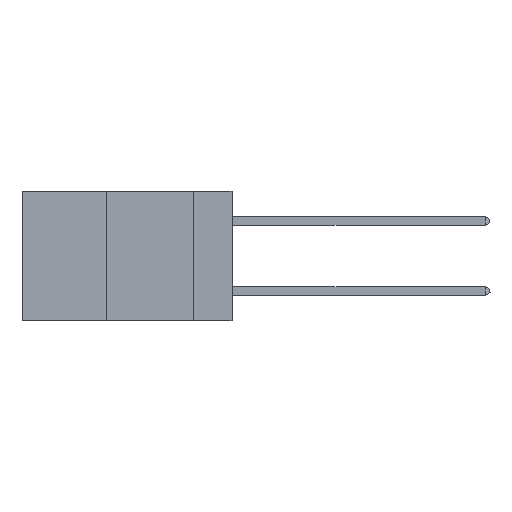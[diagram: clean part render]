
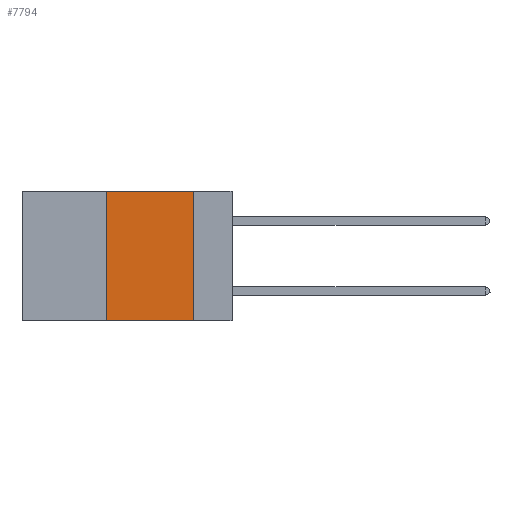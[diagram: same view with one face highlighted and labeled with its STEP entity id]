
A CAD part, left-side view. The second image highlights one B-rep face of the part: STEP entity #7794.
In plain terms, the highlighted planar face has unit normal (-1, 0, 0).
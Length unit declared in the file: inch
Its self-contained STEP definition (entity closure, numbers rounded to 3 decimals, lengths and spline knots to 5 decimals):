
#4075 = VERTEX_POINT ( 'NONE', #21904 ) ;
#4447 = VECTOR ( 'NONE', #21325, 39.37008 ) ;
#6490 = EDGE_CURVE ( 'NONE', #4075, #15165, #25839, .T. ) ;
#7478 = VECTOR ( 'NONE', #22442, 39.37008 ) ;
#7794 = ADVANCED_FACE ( 'NONE', ( #26321 ), #20868, .F. ) ;
#9089 = ORIENTED_EDGE ( 'NONE', *, *, #14328, .T. ) ;
#9822 = CARTESIAN_POINT ( 'NONE',  ( 0., 0.11, -0.37 ) ) ;
#9927 = CARTESIAN_POINT ( 'NONE',  ( 0., 0.11, 0. ) ) ;
#10688 = AXIS2_PLACEMENT_3D ( 'NONE', #18592, #23290, #18900 ) ;
#11420 = CARTESIAN_POINT ( 'NONE',  ( 0., 0.11, 0. ) ) ;
#12205 = LINE ( 'NONE', #24849, #7478 ) ;
#12572 = VECTOR ( 'NONE', #28287, 39.37008 ) ;
#12920 = LINE ( 'NONE', #17652, #14794 ) ;
#13844 = LINE ( 'NONE', #11420, #4447 ) ;
#14042 = ORIENTED_EDGE ( 'NONE', *, *, #24259, .F. ) ;
#14328 = EDGE_CURVE ( 'NONE', #4075, #25190, #12205, .T. ) ;
#14794 = VECTOR ( 'NONE', #29953, 39.37008 ) ;
#14892 = CARTESIAN_POINT ( 'NONE',  ( 0., 0.36, 0. ) ) ;
#15165 = VERTEX_POINT ( 'NONE', #14892 ) ;
#17652 = CARTESIAN_POINT ( 'NONE',  ( 0., 0.6, 0. ) ) ;
#18592 = CARTESIAN_POINT ( 'NONE',  ( 0., 0.6, 0. ) ) ;
#18900 = DIRECTION ( 'NONE',  ( 0., 0., -1. ) ) ;
#20868 = PLANE ( 'NONE',  #10688 ) ;
#20963 = EDGE_LOOP ( 'NONE', ( #14042, #23764, #27486, #9089 ) ) ;
#21325 = DIRECTION ( 'NONE',  ( 0., 0., -1. ) ) ;
#21904 = CARTESIAN_POINT ( 'NONE',  ( 0., 0.36, -0.37 ) ) ;
#22442 = DIRECTION ( 'NONE',  ( 0., -1., 0. ) ) ;
#22722 = VERTEX_POINT ( 'NONE', #9927 ) ;
#23290 = DIRECTION ( 'NONE',  ( 1., 0., 0. ) ) ;
#23764 = ORIENTED_EDGE ( 'NONE', *, *, #30517, .F. ) ;
#24259 = EDGE_CURVE ( 'NONE', #22722, #25190, #13844, .T. ) ;
#24849 = CARTESIAN_POINT ( 'NONE',  ( 0., 0.6, -0.37 ) ) ;
#25190 = VERTEX_POINT ( 'NONE', #9822 ) ;
#25839 = LINE ( 'NONE', #28604, #12572 ) ;
#26321 = FACE_OUTER_BOUND ( 'NONE', #20963, .T. ) ;
#27486 = ORIENTED_EDGE ( 'NONE', *, *, #6490, .F. ) ;
#28287 = DIRECTION ( 'NONE',  ( 0., 0., 1. ) ) ;
#28604 = CARTESIAN_POINT ( 'NONE',  ( 0., 0.36, 0. ) ) ;
#29953 = DIRECTION ( 'NONE',  ( 0., -1., 0. ) ) ;
#30517 = EDGE_CURVE ( 'NONE', #15165, #22722, #12920, .T. ) ;
